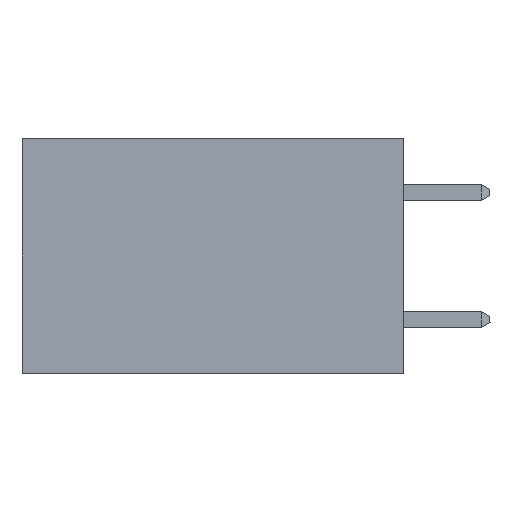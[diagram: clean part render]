
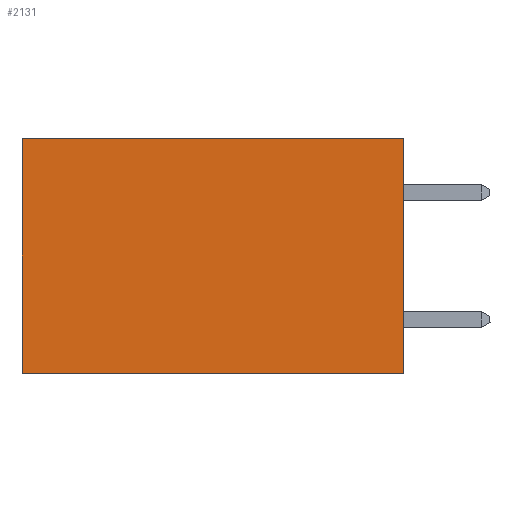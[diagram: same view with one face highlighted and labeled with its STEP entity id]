
A CAD part, left-side view. The second image highlights one B-rep face of the part: STEP entity #2131.
In plain terms, the highlighted planar face has unit normal (-1, 0, 0).
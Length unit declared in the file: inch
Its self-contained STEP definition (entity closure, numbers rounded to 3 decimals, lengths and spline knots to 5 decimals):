
#736 = VERTEX_POINT ( 'NONE', #3850 ) ;
#808 = LINE ( 'NONE', #2709, #13924 ) ;
#832 = VECTOR ( 'NONE', #1294, 39.37008 ) ;
#1294 = DIRECTION ( 'NONE',  ( 0., 0., -1. ) ) ;
#1494 = CARTESIAN_POINT ( 'NONE',  ( 0.2875, 0.6, -0.37 ) ) ;
#1667 = ORIENTED_EDGE ( 'NONE', *, *, #11000, .F. ) ;
#1873 = LINE ( 'NONE', #10414, #10865 ) ;
#2131 = ADVANCED_FACE ( 'NONE', ( #14568 ), #4682, .F. ) ;
#2385 = ORIENTED_EDGE ( 'NONE', *, *, #11161, .T. ) ;
#2709 = CARTESIAN_POINT ( 'NONE',  ( 0.2875, 0., 0. ) ) ;
#3850 = CARTESIAN_POINT ( 'NONE',  ( 0.2875, 0., -0.37 ) ) ;
#4231 = ORIENTED_EDGE ( 'NONE', *, *, #11611, .F. ) ;
#4546 = DIRECTION ( 'NONE',  ( 0., 0., -1. ) ) ;
#4621 = DIRECTION ( 'NONE',  ( 1., 0., 0. ) ) ;
#4682 = PLANE ( 'NONE',  #8003 ) ;
#4758 = LINE ( 'NONE', #15660, #15451 ) ;
#5080 = EDGE_LOOP ( 'NONE', ( #13771, #1667, #4231, #2385 ) ) ;
#5204 = CARTESIAN_POINT ( 'NONE',  ( 0.2875, 0., 0. ) ) ;
#5415 = DIRECTION ( 'NONE',  ( 0., 1., 0. ) ) ;
#6722 = VERTEX_POINT ( 'NONE', #1494 ) ;
#8003 = AXIS2_PLACEMENT_3D ( 'NONE', #5204, #4621, #4546 ) ;
#8258 = DIRECTION ( 'NONE',  ( 0., 1., 0. ) ) ;
#9726 = CARTESIAN_POINT ( 'NONE',  ( 0.2875, 0., 0. ) ) ;
#10346 = DIRECTION ( 'NONE',  ( 0., 0., -1. ) ) ;
#10414 = CARTESIAN_POINT ( 'NONE',  ( 0.2875, 0., -0.37 ) ) ;
#10865 = VECTOR ( 'NONE', #5415, 39.37008 ) ;
#11000 = EDGE_CURVE ( 'NONE', #736, #6722, #1873, .T. ) ;
#11068 = LINE ( 'NONE', #16386, #832 ) ;
#11161 = EDGE_CURVE ( 'NONE', #12200, #16335, #4758, .T. ) ;
#11611 = EDGE_CURVE ( 'NONE', #12200, #736, #808, .T. ) ;
#12200 = VERTEX_POINT ( 'NONE', #9726 ) ;
#13771 = ORIENTED_EDGE ( 'NONE', *, *, #15674, .T. ) ;
#13924 = VECTOR ( 'NONE', #10346, 39.37008 ) ;
#14568 = FACE_OUTER_BOUND ( 'NONE', #5080, .T. ) ;
#15292 = CARTESIAN_POINT ( 'NONE',  ( 0.2875, 0.6, 0. ) ) ;
#15451 = VECTOR ( 'NONE', #8258, 39.37008 ) ;
#15660 = CARTESIAN_POINT ( 'NONE',  ( 0.2875, 0., 0. ) ) ;
#15674 = EDGE_CURVE ( 'NONE', #16335, #6722, #11068, .T. ) ;
#16335 = VERTEX_POINT ( 'NONE', #15292 ) ;
#16386 = CARTESIAN_POINT ( 'NONE',  ( 0.2875, 0.6, 0. ) ) ;
